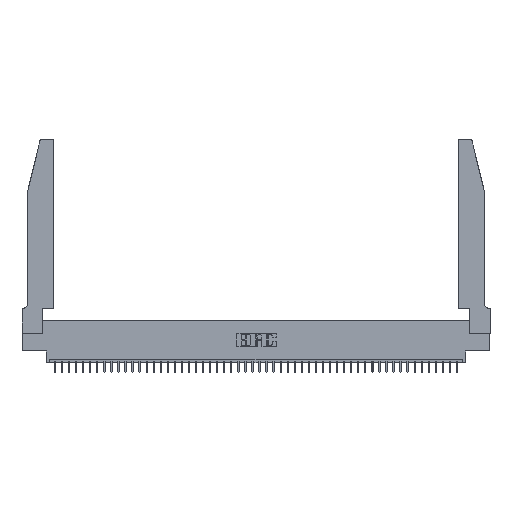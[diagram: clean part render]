
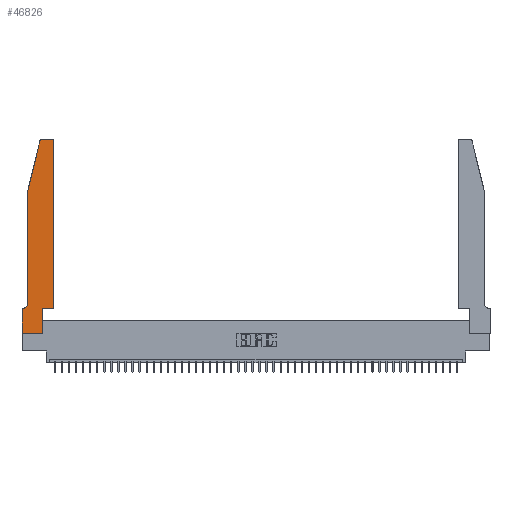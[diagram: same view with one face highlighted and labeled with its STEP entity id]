
A CAD part, top view. The second image highlights one B-rep face of the part: STEP entity #46826.
In plain terms, the highlighted planar face has unit normal (0, 0, 1).
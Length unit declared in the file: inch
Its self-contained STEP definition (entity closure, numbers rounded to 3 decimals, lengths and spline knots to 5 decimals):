
#13 = EDGE_CURVE ( 'NONE', #6229, #6934, #38369, .T. ) ;
#1306 = LINE ( 'NONE', #8664, #4723 ) ;
#1362 = CARTESIAN_POINT ( 'NONE',  ( 0.284, 2.72, 0.37 ) ) ;
#4723 = VECTOR ( 'NONE', #12332, 39.37008 ) ;
#5054 = DIRECTION ( 'NONE',  ( 0., 0., 1. ) ) ;
#5071 = EDGE_CURVE ( 'NONE', #8739, #28199, #18575, .T. ) ;
#5814 = CIRCLE ( 'NONE', #14285, 0.03 ) ;
#5828 = CARTESIAN_POINT ( 'NONE',  ( 0.4505, 0.35, 0.37 ) ) ;
#6068 = AXIS2_PLACEMENT_3D ( 'NONE', #10478, #26135, #41037 ) ;
#6229 = VERTEX_POINT ( 'NONE', #28241 ) ;
#6371 = EDGE_CURVE ( 'NONE', #28199, #6229, #25516, .T. ) ;
#6662 = CARTESIAN_POINT ( 'NONE',  ( 0.4205, 2.75, 0.37 ) ) ;
#6727 = CARTESIAN_POINT ( 'NONE',  ( 0.284, 2.75, 0.37 ) ) ;
#6934 = VERTEX_POINT ( 'NONE', #8080 ) ;
#8080 = CARTESIAN_POINT ( 'NONE',  ( 0.4505, 0.35, 0.37 ) ) ;
#8166 = DIRECTION ( 'NONE',  ( 0., 0., 1. ) ) ;
#8466 = EDGE_CURVE ( 'NONE', #16252, #8739, #33237, .T. ) ;
#8664 = CARTESIAN_POINT ( 'NONE',  ( 0.4505, 0.35, 0.37 ) ) ;
#8739 = VERTEX_POINT ( 'NONE', #13156 ) ;
#9722 = VERTEX_POINT ( 'NONE', #42378 ) ;
#10252 = CARTESIAN_POINT ( 'NONE',  ( 0., 0., 0.37 ) ) ;
#10478 = CARTESIAN_POINT ( 'NONE',  ( 0.0055, 0.42, 0.37 ) ) ;
#11332 = VECTOR ( 'NONE', #20643, 39.37008 ) ;
#12332 = DIRECTION ( 'NONE',  ( 0., 1., 0. ) ) ;
#12752 = CARTESIAN_POINT ( 'NONE',  ( 0.25487, 2.72718, 0.37 ) ) ;
#13156 = CARTESIAN_POINT ( 'NONE',  ( 0., 0., 0.37 ) ) ;
#13787 = CARTESIAN_POINT ( 'NONE',  ( 0.4505, 2.72, 0.37 ) ) ;
#14285 = AXIS2_PLACEMENT_3D ( 'NONE', #36554, #25313, #36099 ) ;
#14641 = ORIENTED_EDGE ( 'NONE', *, *, #23441, .T. ) ;
#14996 = CIRCLE ( 'NONE', #42375, 0.03 ) ;
#15267 = DIRECTION ( 'NONE',  ( 1., 0., 0. ) ) ;
#16252 = VERTEX_POINT ( 'NONE', #38980 ) ;
#16438 = ORIENTED_EDGE ( 'NONE', *, *, #28839, .T. ) ;
#17598 = CARTESIAN_POINT ( 'NONE',  ( 0.2865, 0., 0.37 ) ) ;
#18091 = DIRECTION ( 'NONE',  ( 1., 0., 0. ) ) ;
#18575 = LINE ( 'NONE', #33506, #47733 ) ;
#18829 = ORIENTED_EDGE ( 'NONE', *, *, #39692, .T. ) ;
#19069 = DIRECTION ( 'NONE',  ( -0.239, -0.971, 0. ) ) ;
#19187 = VERTEX_POINT ( 'NONE', #13787 ) ;
#19752 = DIRECTION ( 'NONE',  ( 1., 0., 0. ) ) ;
#20400 = LINE ( 'NONE', #24549, #11332 ) ;
#20643 = DIRECTION ( 'NONE',  ( 0., -1., 0. ) ) ;
#20761 = DIRECTION ( 'NONE',  ( 1., 0., 0. ) ) ;
#23182 = VECTOR ( 'NONE', #20761, 39.37008 ) ;
#23441 = EDGE_CURVE ( 'NONE', #19187, #25235, #5814, .T. ) ;
#23785 = CARTESIAN_POINT ( 'NONE',  ( 0.2605, 2.75, 0.37 ) ) ;
#24359 = ORIENTED_EDGE ( 'NONE', *, *, #6371, .T. ) ;
#24549 = CARTESIAN_POINT ( 'NONE',  ( 0.0755, 2., 0.37 ) ) ;
#25164 = VECTOR ( 'NONE', #25186, 39.37008 ) ;
#25186 = DIRECTION ( 'NONE',  ( 0., -1., 0. ) ) ;
#25235 = VERTEX_POINT ( 'NONE', #6662 ) ;
#25313 = DIRECTION ( 'NONE',  ( 0., 0., 1. ) ) ;
#25435 = VERTEX_POINT ( 'NONE', #12752 ) ;
#25516 = LINE ( 'NONE', #37016, #25768 ) ;
#25768 = VECTOR ( 'NONE', #29410, 39.37008 ) ;
#25954 = AXIS2_PLACEMENT_3D ( 'NONE', #38259, #8166, #15267 ) ;
#26135 = DIRECTION ( 'NONE',  ( 0., 0., -1. ) ) ;
#26649 = LINE ( 'NONE', #29573, #44641 ) ;
#28199 = VERTEX_POINT ( 'NONE', #17598 ) ;
#28241 = CARTESIAN_POINT ( 'NONE',  ( 0.2865, 0.35, 0.37 ) ) ;
#28839 = EDGE_CURVE ( 'NONE', #41483, #9722, #20400, .T. ) ;
#29410 = DIRECTION ( 'NONE',  ( 0., 1., 0. ) ) ;
#29573 = CARTESIAN_POINT ( 'NONE',  ( 0.0755, 2., 0.37 ) ) ;
#29883 = ORIENTED_EDGE ( 'NONE', *, *, #46549, .T. ) ;
#30913 = FACE_OUTER_BOUND ( 'NONE', #36366, .T. ) ;
#31019 = LINE ( 'NONE', #45935, #41464 ) ;
#31109 = LINE ( 'NONE', #23785, #32914 ) ;
#32184 = ORIENTED_EDGE ( 'NONE', *, *, #43682, .T. ) ;
#32914 = VECTOR ( 'NONE', #42113, 39.37008 ) ;
#33237 = LINE ( 'NONE', #10252, #25164 ) ;
#33506 = CARTESIAN_POINT ( 'NONE',  ( 0., 0., 0.37 ) ) ;
#33886 = PLANE ( 'NONE',  #25954 ) ;
#34170 = CARTESIAN_POINT ( 'NONE',  ( 0.0755, 2., 0.37 ) ) ;
#34216 = CIRCLE ( 'NONE', #6068, 0.07 ) ;
#35935 = ORIENTED_EDGE ( 'NONE', *, *, #13, .T. ) ;
#36099 = DIRECTION ( 'NONE',  ( 1., 0., 0. ) ) ;
#36101 = VERTEX_POINT ( 'NONE', #46466 ) ;
#36366 = EDGE_LOOP ( 'NONE', ( #47621, #29883, #43320, #16438, #18829, #32184, #37010, #39734, #24359, #35935, #46558, #14641 ) ) ;
#36554 = CARTESIAN_POINT ( 'NONE',  ( 0.4205, 2.72, 0.37 ) ) ;
#36629 = VERTEX_POINT ( 'NONE', #6727 ) ;
#36949 = EDGE_CURVE ( 'NONE', #6934, #19187, #1306, .T. ) ;
#37010 = ORIENTED_EDGE ( 'NONE', *, *, #8466, .T. ) ;
#37016 = CARTESIAN_POINT ( 'NONE',  ( 0.2865, 0.35, 0.37 ) ) ;
#37487 = EDGE_CURVE ( 'NONE', #25235, #36629, #31109, .T. ) ;
#38259 = CARTESIAN_POINT ( 'NONE',  ( 0., 0.35, 0.37 ) ) ;
#38369 = LINE ( 'NONE', #5828, #23182 ) ;
#38605 = DIRECTION ( 'NONE',  ( -1., 0., 0. ) ) ;
#38980 = CARTESIAN_POINT ( 'NONE',  ( 0., 0.35, 0.37 ) ) ;
#39692 = EDGE_CURVE ( 'NONE', #9722, #36101, #34216, .T. ) ;
#39734 = ORIENTED_EDGE ( 'NONE', *, *, #5071, .T. ) ;
#41037 = DIRECTION ( 'NONE',  ( -1., 0., 0. ) ) ;
#41464 = VECTOR ( 'NONE', #38605, 39.37008 ) ;
#41483 = VERTEX_POINT ( 'NONE', #34170 ) ;
#42113 = DIRECTION ( 'NONE',  ( -1., 0., 0. ) ) ;
#42375 = AXIS2_PLACEMENT_3D ( 'NONE', #1362, #5054, #19752 ) ;
#42378 = CARTESIAN_POINT ( 'NONE',  ( 0.0755, 0.42, 0.37 ) ) ;
#43320 = ORIENTED_EDGE ( 'NONE', *, *, #45907, .T. ) ;
#43682 = EDGE_CURVE ( 'NONE', #36101, #16252, #31019, .T. ) ;
#44641 = VECTOR ( 'NONE', #19069, 39.37008 ) ;
#45907 = EDGE_CURVE ( 'NONE', #25435, #41483, #26649, .T. ) ;
#45935 = CARTESIAN_POINT ( 'NONE',  ( 0.0755, 0.35, 0.37 ) ) ;
#46466 = CARTESIAN_POINT ( 'NONE',  ( 0.0055, 0.35, 0.37 ) ) ;
#46549 = EDGE_CURVE ( 'NONE', #36629, #25435, #14996, .T. ) ;
#46558 = ORIENTED_EDGE ( 'NONE', *, *, #36949, .T. ) ;
#46826 = ADVANCED_FACE ( 'NONE', ( #30913 ), #33886, .T. ) ;
#47621 = ORIENTED_EDGE ( 'NONE', *, *, #37487, .T. ) ;
#47733 = VECTOR ( 'NONE', #18091, 39.37008 ) ;
